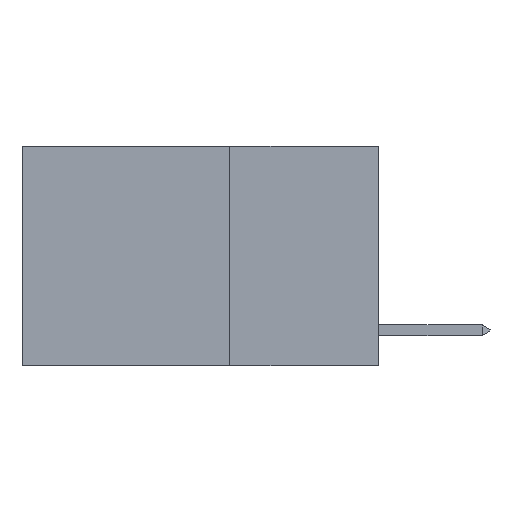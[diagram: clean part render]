
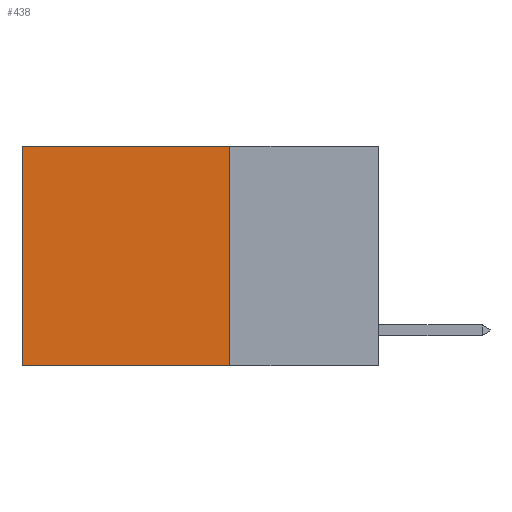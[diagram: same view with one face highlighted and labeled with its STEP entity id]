
A CAD part, left-side view. The second image highlights one B-rep face of the part: STEP entity #438.
In plain terms, the highlighted planar face has unit normal (-1, 0, 0).
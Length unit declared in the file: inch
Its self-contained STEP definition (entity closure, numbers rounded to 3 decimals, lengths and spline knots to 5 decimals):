
#438 = ADVANCED_FACE ( 'NONE', ( #9415 ), #13919, .F. ) ;
#849 = ORIENTED_EDGE ( 'NONE', *, *, #11545, .T. ) ;
#887 = LINE ( 'NONE', #6767, #10366 ) ;
#983 = DIRECTION ( 'NONE',  ( 0., 1., 0. ) ) ;
#1180 = VECTOR ( 'NONE', #11691, 39.37008 ) ;
#1816 = EDGE_CURVE ( 'NONE', #5386, #6388, #887, .T. ) ;
#1862 = CARTESIAN_POINT ( 'NONE',  ( 0.2625, 0.25, 0. ) ) ;
#2642 = EDGE_LOOP ( 'NONE', ( #849, #3678, #3365, #7967 ) ) ;
#3365 = ORIENTED_EDGE ( 'NONE', *, *, #19221, .F. ) ;
#3678 = ORIENTED_EDGE ( 'NONE', *, *, #1816, .F. ) ;
#5386 = VERTEX_POINT ( 'NONE', #14996 ) ;
#6388 = VERTEX_POINT ( 'NONE', #6892 ) ;
#6767 = CARTESIAN_POINT ( 'NONE',  ( 0.2625, 0.25, -0.37 ) ) ;
#6772 = DIRECTION ( 'NONE',  ( 0., 1., 0. ) ) ;
#6892 = CARTESIAN_POINT ( 'NONE',  ( 0.2625, 0.6, -0.37 ) ) ;
#7071 = LINE ( 'NONE', #17217, #10057 ) ;
#7072 = CARTESIAN_POINT ( 'NONE',  ( 0.2625, 0.6, 0. ) ) ;
#7563 = DIRECTION ( 'NONE',  ( 0., 0., -1. ) ) ;
#7967 = ORIENTED_EDGE ( 'NONE', *, *, #8233, .T. ) ;
#8233 = EDGE_CURVE ( 'NONE', #13636, #9459, #7071, .T. ) ;
#9415 = FACE_OUTER_BOUND ( 'NONE', #2642, .T. ) ;
#9459 = VERTEX_POINT ( 'NONE', #7072 ) ;
#10057 = VECTOR ( 'NONE', #6772, 39.37008 ) ;
#10080 = AXIS2_PLACEMENT_3D ( 'NONE', #1862, #10897, #7563 ) ;
#10366 = VECTOR ( 'NONE', #983, 39.37008 ) ;
#10897 = DIRECTION ( 'NONE',  ( 1., 0., 0. ) ) ;
#11545 = EDGE_CURVE ( 'NONE', #9459, #6388, #12717, .T. ) ;
#11691 = DIRECTION ( 'NONE',  ( 0., 0., -1. ) ) ;
#12717 = LINE ( 'NONE', #15921, #18860 ) ;
#12735 = CARTESIAN_POINT ( 'NONE',  ( 0.2625, 0.25, 0. ) ) ;
#13636 = VERTEX_POINT ( 'NONE', #12735 ) ;
#13919 = PLANE ( 'NONE',  #10080 ) ;
#14996 = CARTESIAN_POINT ( 'NONE',  ( 0.2625, 0.25, -0.37 ) ) ;
#15821 = DIRECTION ( 'NONE',  ( 0., 0., -1. ) ) ;
#15921 = CARTESIAN_POINT ( 'NONE',  ( 0.2625, 0.6, 0. ) ) ;
#17217 = CARTESIAN_POINT ( 'NONE',  ( 0.2625, 0.25, 0. ) ) ;
#17631 = CARTESIAN_POINT ( 'NONE',  ( 0.2625, 0.25, 0. ) ) ;
#18860 = VECTOR ( 'NONE', #15821, 39.37008 ) ;
#18906 = LINE ( 'NONE', #17631, #1180 ) ;
#19221 = EDGE_CURVE ( 'NONE', #13636, #5386, #18906, .T. ) ;
